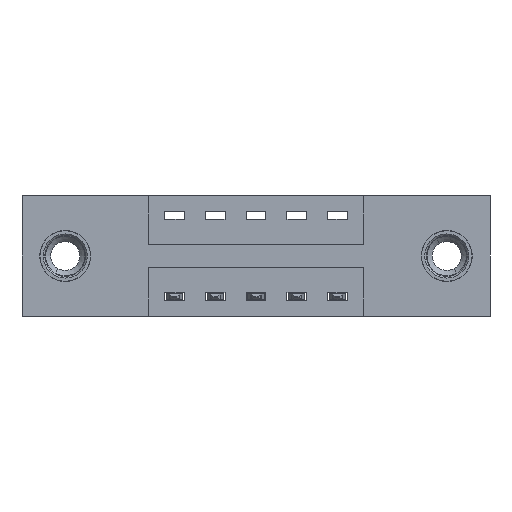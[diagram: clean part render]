
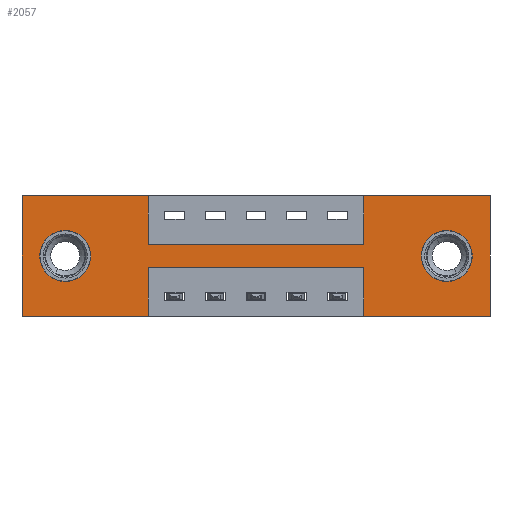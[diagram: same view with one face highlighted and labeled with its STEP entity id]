
A CAD part, front view. The second image highlights one B-rep face of the part: STEP entity #2057.
In plain terms, the highlighted planar face has unit normal (0, -1, 0).
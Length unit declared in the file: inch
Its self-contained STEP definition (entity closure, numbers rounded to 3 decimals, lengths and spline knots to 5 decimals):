
#157 = FACE_OUTER_BOUND ( 'NONE', #8537, .T. ) ;
#186 = CARTESIAN_POINT ( 'NONE',  ( 0., 0., 0. ) ) ;
#209 = CARTESIAN_POINT ( 'NONE',  ( 0.3875, 0., 0. ) ) ;
#328 = ORIENTED_EDGE ( 'NONE', *, *, #9420, .F. ) ;
#424 = DIRECTION ( 'NONE',  ( 0., 1., 0. ) ) ;
#485 = VERTEX_POINT ( 'NONE', #6300 ) ;
#549 = VERTEX_POINT ( 'NONE', #10353 ) ;
#741 = CARTESIAN_POINT ( 'NONE',  ( 0.3875, 0., -0.15 ) ) ;
#745 = ORIENTED_EDGE ( 'NONE', *, *, #3101, .F. ) ;
#848 = VERTEX_POINT ( 'NONE', #10046 ) ;
#935 = VERTEX_POINT ( 'NONE', #9266 ) ;
#985 = LINE ( 'NONE', #186, #3332 ) ;
#998 = DIRECTION ( 'NONE',  ( -1., 0., 0. ) ) ;
#1057 = LINE ( 'NONE', #8564, #7141 ) ;
#1150 = DIRECTION ( 'NONE',  ( 0., 1., 0. ) ) ;
#1176 = DIRECTION ( 'NONE',  ( 0., 0., -1. ) ) ;
#1240 = ORIENTED_EDGE ( 'NONE', *, *, #5377, .T. ) ;
#1453 = AXIS2_PLACEMENT_3D ( 'NONE', #10366, #424, #2475 ) ;
#1589 = CARTESIAN_POINT ( 'NONE',  ( 0., 0., -0.37 ) ) ;
#1597 = DIRECTION ( 'NONE',  ( 0., 0., -1. ) ) ;
#1799 = ORIENTED_EDGE ( 'NONE', *, *, #9002, .F. ) ;
#1867 = DIRECTION ( 'NONE',  ( -1., 0., 0. ) ) ;
#1886 = CIRCLE ( 'NONE', #9368, 0.078 ) ;
#1900 = CARTESIAN_POINT ( 'NONE',  ( 0.3875, 0., -0.22 ) ) ;
#2025 = VERTEX_POINT ( 'NONE', #6582 ) ;
#2057 = ADVANCED_FACE ( 'NONE', ( #2671, #6710, #157 ), #12562, .T. ) ;
#2079 = LINE ( 'NONE', #2212, #5664 ) ;
#2212 = CARTESIAN_POINT ( 'NONE',  ( 1.0475, 0., -0.37 ) ) ;
#2418 = ORIENTED_EDGE ( 'NONE', *, *, #9870, .F. ) ;
#2475 = DIRECTION ( 'NONE',  ( 0., 0., -1. ) ) ;
#2521 = ORIENTED_EDGE ( 'NONE', *, *, #6520, .T. ) ;
#2620 = VECTOR ( 'NONE', #1867, 39.37008 ) ;
#2671 = FACE_BOUND ( 'NONE', #6777, .T. ) ;
#2757 = VECTOR ( 'NONE', #1597, 39.37008 ) ;
#2780 = ORIENTED_EDGE ( 'NONE', *, *, #8392, .F. ) ;
#3070 = CARTESIAN_POINT ( 'NONE',  ( 0., 0., -0.37 ) ) ;
#3091 = LINE ( 'NONE', #1900, #2620 ) ;
#3101 = EDGE_CURVE ( 'NONE', #10898, #6978, #1057, .T. ) ;
#3103 = VECTOR ( 'NONE', #5821, 39.37008 ) ;
#3168 = CARTESIAN_POINT ( 'NONE',  ( 0.1325, 0., -0.185 ) ) ;
#3234 = LINE ( 'NONE', #3968, #8212 ) ;
#3268 = EDGE_CURVE ( 'NONE', #6978, #11364, #9648, .T. ) ;
#3275 = EDGE_CURVE ( 'NONE', #7920, #10898, #6667, .T. ) ;
#3332 = VECTOR ( 'NONE', #4241, 39.37008 ) ;
#3367 = CARTESIAN_POINT ( 'NONE',  ( 1.435, 0., -0.37 ) ) ;
#3466 = CIRCLE ( 'NONE', #1453, 0.078 ) ;
#3470 = EDGE_CURVE ( 'NONE', #848, #12497, #3091, .T. ) ;
#3553 = EDGE_CURVE ( 'NONE', #12140, #2025, #7593, .T. ) ;
#3620 = EDGE_CURVE ( 'NONE', #8893, #3665, #3234, .T. ) ;
#3665 = VERTEX_POINT ( 'NONE', #3367 ) ;
#3685 = CARTESIAN_POINT ( 'NONE',  ( 1.0475, 0., 0. ) ) ;
#3761 = ORIENTED_EDGE ( 'NONE', *, *, #3275, .F. ) ;
#3765 = DIRECTION ( 'NONE',  ( 0., -1., 0. ) ) ;
#3968 = CARTESIAN_POINT ( 'NONE',  ( 1.435, 0., 0. ) ) ;
#4074 = DIRECTION ( 'NONE',  ( 0., 1., 0. ) ) ;
#4204 = VECTOR ( 'NONE', #998, 39.37008 ) ;
#4241 = DIRECTION ( 'NONE',  ( 0., 0., 1. ) ) ;
#4502 = VECTOR ( 'NONE', #7049, 39.37008 ) ;
#4685 = CARTESIAN_POINT ( 'NONE',  ( 1.0475, 0., 0. ) ) ;
#4717 = DIRECTION ( 'NONE',  ( 0., 0., -1. ) ) ;
#4803 = AXIS2_PLACEMENT_3D ( 'NONE', #4980, #7161, #1176 ) ;
#4874 = ORIENTED_EDGE ( 'NONE', *, *, #10862, .F. ) ;
#4980 = CARTESIAN_POINT ( 'NONE',  ( 1.3025, 0., -0.185 ) ) ;
#5067 = DIRECTION ( 'NONE',  ( 0., 0., 1. ) ) ;
#5377 = EDGE_CURVE ( 'NONE', #6229, #549, #8370, .T. ) ;
#5470 = DIRECTION ( 'NONE',  ( 1., 0., 0. ) ) ;
#5664 = VECTOR ( 'NONE', #11307, 39.37008 ) ;
#5821 = DIRECTION ( 'NONE',  ( 0., 0., -1. ) ) ;
#6229 = VERTEX_POINT ( 'NONE', #12535 ) ;
#6300 = CARTESIAN_POINT ( 'NONE',  ( 0., 0., 0. ) ) ;
#6345 = CARTESIAN_POINT ( 'NONE',  ( 1.0475, 0., -0.37 ) ) ;
#6520 = EDGE_CURVE ( 'NONE', #2025, #12140, #3466, .T. ) ;
#6576 = ORIENTED_EDGE ( 'NONE', *, *, #7397, .F. ) ;
#6582 = CARTESIAN_POINT ( 'NONE',  ( 1.3025, 0., -0.263 ) ) ;
#6634 = ORIENTED_EDGE ( 'NONE', *, *, #3553, .T. ) ;
#6667 = LINE ( 'NONE', #12758, #3103 ) ;
#6710 = FACE_BOUND ( 'NONE', #9102, .T. ) ;
#6724 = DIRECTION ( 'NONE',  ( 0., 0., 1. ) ) ;
#6725 = CARTESIAN_POINT ( 'NONE',  ( 0.3875, 0., -0.37 ) ) ;
#6777 = EDGE_LOOP ( 'NONE', ( #6634, #2521 ) ) ;
#6978 = VERTEX_POINT ( 'NONE', #8730 ) ;
#7049 = DIRECTION ( 'NONE',  ( 1., 0., 0. ) ) ;
#7141 = VECTOR ( 'NONE', #5470, 39.37008 ) ;
#7161 = DIRECTION ( 'NONE',  ( 0., 1., 0. ) ) ;
#7192 = CARTESIAN_POINT ( 'NONE',  ( 1.435, 0., 0. ) ) ;
#7397 = EDGE_CURVE ( 'NONE', #935, #485, #985, .T. ) ;
#7404 = ORIENTED_EDGE ( 'NONE', *, *, #3268, .F. ) ;
#7418 = LINE ( 'NONE', #6725, #2757 ) ;
#7425 = ORIENTED_EDGE ( 'NONE', *, *, #11468, .T. ) ;
#7593 = CIRCLE ( 'NONE', #4803, 0.078 ) ;
#7617 = CARTESIAN_POINT ( 'NONE',  ( 0., 0., 0. ) ) ;
#7730 = EDGE_CURVE ( 'NONE', #11094, #935, #7961, .T. ) ;
#7767 = CARTESIAN_POINT ( 'NONE',  ( 0.3875, 0., -0.37 ) ) ;
#7832 = DIRECTION ( 'NONE',  ( -1., 0., 0. ) ) ;
#7857 = ORIENTED_EDGE ( 'NONE', *, *, #7730, .F. ) ;
#7920 = VERTEX_POINT ( 'NONE', #209 ) ;
#7961 = LINE ( 'NONE', #8530, #8901 ) ;
#8073 = ORIENTED_EDGE ( 'NONE', *, *, #3620, .F. ) ;
#8212 = VECTOR ( 'NONE', #11012, 39.37008 ) ;
#8370 = CIRCLE ( 'NONE', #11857, 0.078 ) ;
#8392 = EDGE_CURVE ( 'NONE', #12497, #11094, #7418, .T. ) ;
#8521 = AXIS2_PLACEMENT_3D ( 'NONE', #1589, #3765, #4717 ) ;
#8530 = CARTESIAN_POINT ( 'NONE',  ( 0., 0., -0.37 ) ) ;
#8537 = EDGE_LOOP ( 'NONE', ( #2780, #11685, #328, #2418, #8073, #4874, #7404, #745, #3761, #1799, #6576, #7857 ) ) ;
#8564 = CARTESIAN_POINT ( 'NONE',  ( 0.3875, 0., -0.15 ) ) ;
#8730 = CARTESIAN_POINT ( 'NONE',  ( 1.0475, 0., -0.15 ) ) ;
#8893 = VERTEX_POINT ( 'NONE', #7192 ) ;
#8901 = VECTOR ( 'NONE', #7832, 39.37008 ) ;
#9002 = EDGE_CURVE ( 'NONE', #485, #7920, #12506, .T. ) ;
#9102 = EDGE_LOOP ( 'NONE', ( #7425, #1240 ) ) ;
#9266 = CARTESIAN_POINT ( 'NONE',  ( 0., 0., -0.37 ) ) ;
#9368 = AXIS2_PLACEMENT_3D ( 'NONE', #3168, #4074, #5067 ) ;
#9420 = EDGE_CURVE ( 'NONE', #11534, #848, #2079, .T. ) ;
#9594 = DIRECTION ( 'NONE',  ( 1., 0., 0. ) ) ;
#9648 = LINE ( 'NONE', #4685, #12014 ) ;
#9870 = EDGE_CURVE ( 'NONE', #3665, #11534, #10159, .T. ) ;
#10046 = CARTESIAN_POINT ( 'NONE',  ( 1.0475, 0., -0.22 ) ) ;
#10121 = CARTESIAN_POINT ( 'NONE',  ( 0.3875, 0., -0.22 ) ) ;
#10159 = LINE ( 'NONE', #3070, #4204 ) ;
#10353 = CARTESIAN_POINT ( 'NONE',  ( 0.1325, 0., -0.107 ) ) ;
#10366 = CARTESIAN_POINT ( 'NONE',  ( 1.3025, 0., -0.185 ) ) ;
#10652 = CARTESIAN_POINT ( 'NONE',  ( 1.3025, 0., -0.107 ) ) ;
#10862 = EDGE_CURVE ( 'NONE', #11364, #8893, #11112, .T. ) ;
#10898 = VERTEX_POINT ( 'NONE', #741 ) ;
#10996 = DIRECTION ( 'NONE',  ( 0., 0., 1. ) ) ;
#11012 = DIRECTION ( 'NONE',  ( 0., 0., -1. ) ) ;
#11094 = VERTEX_POINT ( 'NONE', #7767 ) ;
#11112 = LINE ( 'NONE', #7617, #11262 ) ;
#11167 = CARTESIAN_POINT ( 'NONE',  ( 0.1325, 0., -0.185 ) ) ;
#11262 = VECTOR ( 'NONE', #9594, 39.37008 ) ;
#11307 = DIRECTION ( 'NONE',  ( 0., 0., 1. ) ) ;
#11364 = VERTEX_POINT ( 'NONE', #3685 ) ;
#11468 = EDGE_CURVE ( 'NONE', #549, #6229, #1886, .T. ) ;
#11534 = VERTEX_POINT ( 'NONE', #6345 ) ;
#11685 = ORIENTED_EDGE ( 'NONE', *, *, #3470, .F. ) ;
#11857 = AXIS2_PLACEMENT_3D ( 'NONE', #11167, #1150, #10996 ) ;
#12014 = VECTOR ( 'NONE', #6724, 39.37008 ) ;
#12139 = CARTESIAN_POINT ( 'NONE',  ( 0., 0., 0. ) ) ;
#12140 = VERTEX_POINT ( 'NONE', #10652 ) ;
#12497 = VERTEX_POINT ( 'NONE', #10121 ) ;
#12506 = LINE ( 'NONE', #12139, #4502 ) ;
#12535 = CARTESIAN_POINT ( 'NONE',  ( 0.1325, 0., -0.263 ) ) ;
#12562 = PLANE ( 'NONE',  #8521 ) ;
#12758 = CARTESIAN_POINT ( 'NONE',  ( 0.3875, 0., 0. ) ) ;
